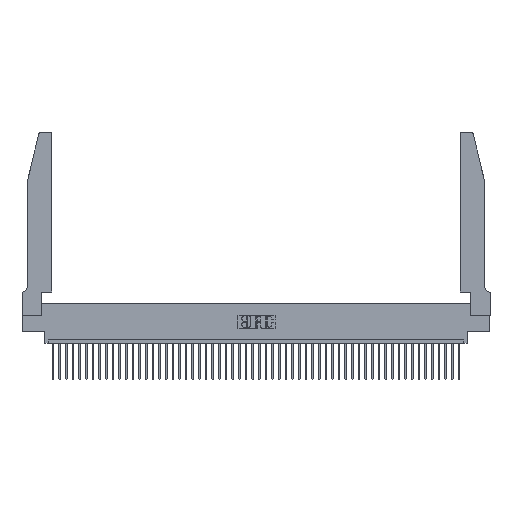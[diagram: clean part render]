
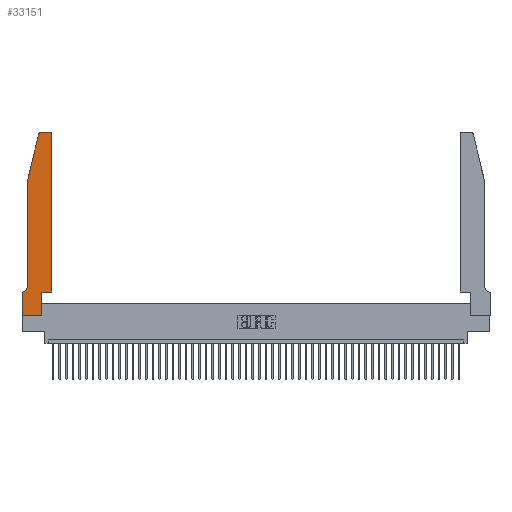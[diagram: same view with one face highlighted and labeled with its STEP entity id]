
A CAD part, top view. The second image highlights one B-rep face of the part: STEP entity #33151.
In plain terms, the highlighted planar face has unit normal (0, 0, 1).
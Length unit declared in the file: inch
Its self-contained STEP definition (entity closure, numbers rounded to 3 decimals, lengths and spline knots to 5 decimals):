
#937 = DIRECTION ( 'NONE',  ( 0., 0., 1. ) ) ;
#1137 = DIRECTION ( 'NONE',  ( 0., 0., -1. ) ) ;
#1305 = EDGE_CURVE ( 'NONE', #42625, #22148, #4845, .T. ) ;
#2131 = VECTOR ( 'NONE', #21804, 39.37008 ) ;
#3153 = DIRECTION ( 'NONE',  ( 0., 0., 1. ) ) ;
#3682 = ORIENTED_EDGE ( 'NONE', *, *, #47803, .T. ) ;
#4845 = LINE ( 'NONE', #48080, #48594 ) ;
#5663 = CARTESIAN_POINT ( 'NONE',  ( 0.0055, 0.35, 0.37 ) ) ;
#6375 = CARTESIAN_POINT ( 'NONE',  ( 0.284, 2.72, 0.37 ) ) ;
#6877 = DIRECTION ( 'NONE',  ( 1., 0., 0. ) ) ;
#7388 = LINE ( 'NONE', #12242, #12042 ) ;
#8000 = CIRCLE ( 'NONE', #10798, 0.03 ) ;
#8570 = ORIENTED_EDGE ( 'NONE', *, *, #1305, .T. ) ;
#8633 = VECTOR ( 'NONE', #43654, 39.37008 ) ;
#8725 = CARTESIAN_POINT ( 'NONE',  ( 0., 0.35, 0.37 ) ) ;
#9486 = EDGE_CURVE ( 'NONE', #18836, #42250, #47019, .T. ) ;
#9676 = EDGE_CURVE ( 'NONE', #42271, #44865, #8000, .T. ) ;
#10798 = AXIS2_PLACEMENT_3D ( 'NONE', #6375, #29000, #6877 ) ;
#11087 = LINE ( 'NONE', #17971, #2131 ) ;
#11111 = ORIENTED_EDGE ( 'NONE', *, *, #27516, .T. ) ;
#11877 = LINE ( 'NONE', #24183, #27866 ) ;
#12042 = VECTOR ( 'NONE', #46236, 39.37008 ) ;
#12242 = CARTESIAN_POINT ( 'NONE',  ( 0.2865, 0.35, 0.37 ) ) ;
#12358 = VECTOR ( 'NONE', #13128, 39.37008 ) ;
#12568 = VERTEX_POINT ( 'NONE', #29878 ) ;
#12625 = ORIENTED_EDGE ( 'NONE', *, *, #44201, .T. ) ;
#13128 = DIRECTION ( 'NONE',  ( -1., 0., 0. ) ) ;
#13286 = AXIS2_PLACEMENT_3D ( 'NONE', #35072, #1137, #46745 ) ;
#13343 = EDGE_CURVE ( 'NONE', #12568, #24682, #19816, .T. ) ;
#13383 = VERTEX_POINT ( 'NONE', #21175 ) ;
#14118 = FACE_OUTER_BOUND ( 'NONE', #45794, .T. ) ;
#14400 = PLANE ( 'NONE',  #33673 ) ;
#15111 = VERTEX_POINT ( 'NONE', #48427 ) ;
#16714 = DIRECTION ( 'NONE',  ( 0., 1., 0. ) ) ;
#17268 = CARTESIAN_POINT ( 'NONE',  ( 0.2605, 2.75, 0.37 ) ) ;
#17638 = LINE ( 'NONE', #17268, #45439 ) ;
#17971 = CARTESIAN_POINT ( 'NONE',  ( 0.0755, 2., 0.37 ) ) ;
#18836 = VERTEX_POINT ( 'NONE', #39714 ) ;
#19816 = LINE ( 'NONE', #28806, #8633 ) ;
#20396 = CARTESIAN_POINT ( 'NONE',  ( 0., 0., 0.37 ) ) ;
#20573 = DIRECTION ( 'NONE',  ( 1., 0., 0. ) ) ;
#21175 = CARTESIAN_POINT ( 'NONE',  ( 0.2865, 0., 0.37 ) ) ;
#21736 = VECTOR ( 'NONE', #20573, 39.37008 ) ;
#21804 = DIRECTION ( 'NONE',  ( -0.239, -0.971, 0. ) ) ;
#22148 = VERTEX_POINT ( 'NONE', #40595 ) ;
#24087 = EDGE_CURVE ( 'NONE', #24682, #25016, #41876, .T. ) ;
#24183 = CARTESIAN_POINT ( 'NONE',  ( 0.4505, 0.35, 0.37 ) ) ;
#24540 = CARTESIAN_POINT ( 'NONE',  ( 0.0755, 0.35, 0.37 ) ) ;
#24682 = VERTEX_POINT ( 'NONE', #48008 ) ;
#24752 = CARTESIAN_POINT ( 'NONE',  ( 0.4505, 2.72, 0.37 ) ) ;
#25016 = VERTEX_POINT ( 'NONE', #5663 ) ;
#25090 = DIRECTION ( 'NONE',  ( -1., 0., 0. ) ) ;
#25827 = VECTOR ( 'NONE', #33363, 39.37008 ) ;
#27516 = EDGE_CURVE ( 'NONE', #37953, #15111, #35255, .T. ) ;
#27751 = DIRECTION ( 'NONE',  ( 1., 0., 0. ) ) ;
#27866 = VECTOR ( 'NONE', #16714, 39.37008 ) ;
#28806 = CARTESIAN_POINT ( 'NONE',  ( 0.0755, 2., 0.37 ) ) ;
#29000 = DIRECTION ( 'NONE',  ( 0., 0., 1. ) ) ;
#29878 = CARTESIAN_POINT ( 'NONE',  ( 0.0755, 2., 0.37 ) ) ;
#30649 = EDGE_CURVE ( 'NONE', #25016, #42625, #42582, .T. ) ;
#32437 = AXIS2_PLACEMENT_3D ( 'NONE', #42633, #937, #27751 ) ;
#32746 = CARTESIAN_POINT ( 'NONE',  ( 0.284, 2.75, 0.37 ) ) ;
#33151 = ADVANCED_FACE ( 'NONE', ( #14118 ), #14400, .T. ) ;
#33363 = DIRECTION ( 'NONE',  ( 1., 0., 0. ) ) ;
#33673 = AXIS2_PLACEMENT_3D ( 'NONE', #37561, #3153, #48539 ) ;
#34794 = LINE ( 'NONE', #20396, #21736 ) ;
#35072 = CARTESIAN_POINT ( 'NONE',  ( 0.0055, 0.42, 0.37 ) ) ;
#35255 = CIRCLE ( 'NONE', #32437, 0.03 ) ;
#36710 = ORIENTED_EDGE ( 'NONE', *, *, #30649, .T. ) ;
#37066 = ORIENTED_EDGE ( 'NONE', *, *, #24087, .T. ) ;
#37071 = ORIENTED_EDGE ( 'NONE', *, *, #9676, .T. ) ;
#37477 = ORIENTED_EDGE ( 'NONE', *, *, #9486, .T. ) ;
#37561 = CARTESIAN_POINT ( 'NONE',  ( 0., 0.35, 0.37 ) ) ;
#37953 = VERTEX_POINT ( 'NONE', #24752 ) ;
#38385 = DIRECTION ( 'NONE',  ( 0., -1., 0. ) ) ;
#39647 = CARTESIAN_POINT ( 'NONE',  ( 0.25487, 2.72718, 0.37 ) ) ;
#39714 = CARTESIAN_POINT ( 'NONE',  ( 0.2865, 0.35, 0.37 ) ) ;
#40020 = CARTESIAN_POINT ( 'NONE',  ( 0.4505, 0.35, 0.37 ) ) ;
#40484 = CARTESIAN_POINT ( 'NONE',  ( 0.4505, 0.35, 0.37 ) ) ;
#40595 = CARTESIAN_POINT ( 'NONE',  ( 0., 0., 0.37 ) ) ;
#40933 = EDGE_CURVE ( 'NONE', #22148, #13383, #34794, .T. ) ;
#41876 = CIRCLE ( 'NONE', #13286, 0.07 ) ;
#42192 = EDGE_CURVE ( 'NONE', #44865, #12568, #11087, .T. ) ;
#42250 = VERTEX_POINT ( 'NONE', #40020 ) ;
#42271 = VERTEX_POINT ( 'NONE', #32746 ) ;
#42474 = ORIENTED_EDGE ( 'NONE', *, *, #46545, .T. ) ;
#42582 = LINE ( 'NONE', #24540, #12358 ) ;
#42625 = VERTEX_POINT ( 'NONE', #8725 ) ;
#42633 = CARTESIAN_POINT ( 'NONE',  ( 0.4205, 2.72, 0.37 ) ) ;
#43654 = DIRECTION ( 'NONE',  ( 0., -1., 0. ) ) ;
#43945 = ORIENTED_EDGE ( 'NONE', *, *, #40933, .T. ) ;
#44201 = EDGE_CURVE ( 'NONE', #13383, #18836, #7388, .T. ) ;
#44865 = VERTEX_POINT ( 'NONE', #39647 ) ;
#45377 = ORIENTED_EDGE ( 'NONE', *, *, #42192, .T. ) ;
#45439 = VECTOR ( 'NONE', #25090, 39.37008 ) ;
#45794 = EDGE_LOOP ( 'NONE', ( #3682, #37071, #45377, #45908, #37066, #36710, #8570, #43945, #12625, #37477, #42474, #11111 ) ) ;
#45908 = ORIENTED_EDGE ( 'NONE', *, *, #13343, .T. ) ;
#46236 = DIRECTION ( 'NONE',  ( 0., 1., 0. ) ) ;
#46545 = EDGE_CURVE ( 'NONE', #42250, #37953, #11877, .T. ) ;
#46745 = DIRECTION ( 'NONE',  ( -1., 0., 0. ) ) ;
#47019 = LINE ( 'NONE', #40484, #25827 ) ;
#47803 = EDGE_CURVE ( 'NONE', #15111, #42271, #17638, .T. ) ;
#48008 = CARTESIAN_POINT ( 'NONE',  ( 0.0755, 0.42, 0.37 ) ) ;
#48080 = CARTESIAN_POINT ( 'NONE',  ( 0., 0., 0.37 ) ) ;
#48427 = CARTESIAN_POINT ( 'NONE',  ( 0.4205, 2.75, 0.37 ) ) ;
#48539 = DIRECTION ( 'NONE',  ( 1., 0., 0. ) ) ;
#48594 = VECTOR ( 'NONE', #38385, 39.37008 ) ;
